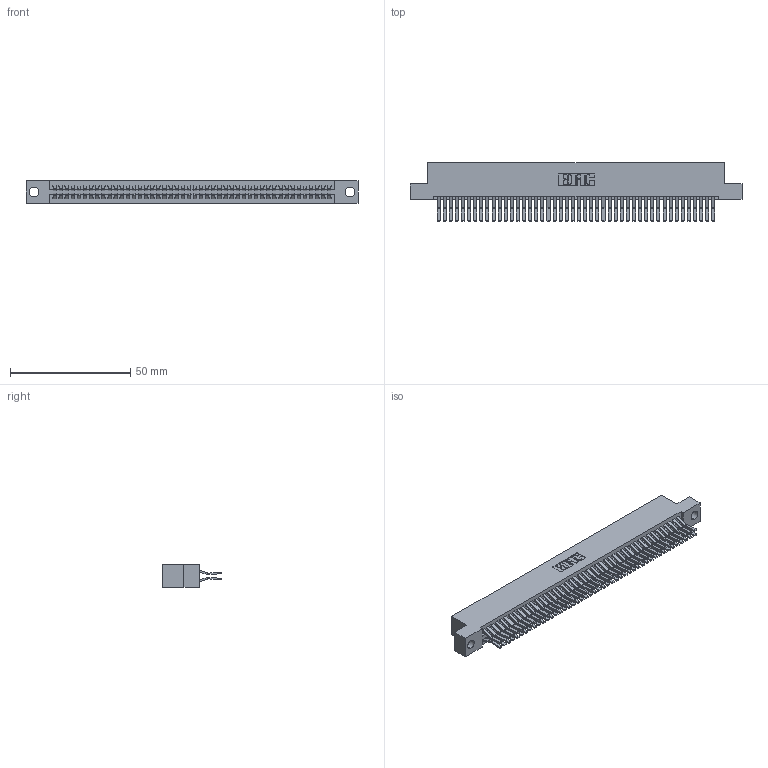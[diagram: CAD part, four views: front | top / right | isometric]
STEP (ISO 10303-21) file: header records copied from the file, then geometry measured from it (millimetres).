
FILE_DESCRIPTION (( 'STEP AP203' ), '1' );
FILE_NAME ('345-092-560-204.STEP', '2018-10-04T22:49:49', ( '' ), ( '' ), 'SwSTEP 2.0', 'SolidWorks 2016', '' );
FILE_SCHEMA (( 'CONFIG_CONTROL_DESIGN' ));
Length unit declared in the file: inch
Products named in the file (3): 345-092-560-204; 345-292-001_560 Tail; 345 Part_Flush Mounting Lugs - 0.156 Dia-TH
Assembly tree (93 placements, depth 2):
  345-092-560-204
    345 Part_Flush Mounting Lugs - 0.156 Dia-TH
    345-292-001_560 Tail  x92
Bounding box: 138.05 x 24.45 x 9.4 mm (x, y, z)
Volume: 13962.5 mm3; surface area: 22082.5 mm2
Topology: 93 solids, 93 shells, 4910 faces, 14601 edges, 9610 vertices
Faces by surface type: plane 3116, cylinder 1794
Entity records: 35645 total; most frequent: CARTESIAN_POINT 5972, ORIENTED_EDGE 5906, DIRECTION 5265, EDGE_CURVE 2953, VECTOR 2633, LINE 2633, VERTEX_POINT 1966, AXIS2_PLACEMENT_3D 1316
